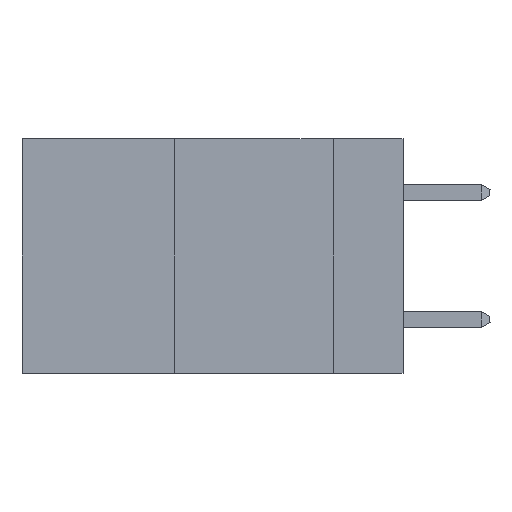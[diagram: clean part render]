
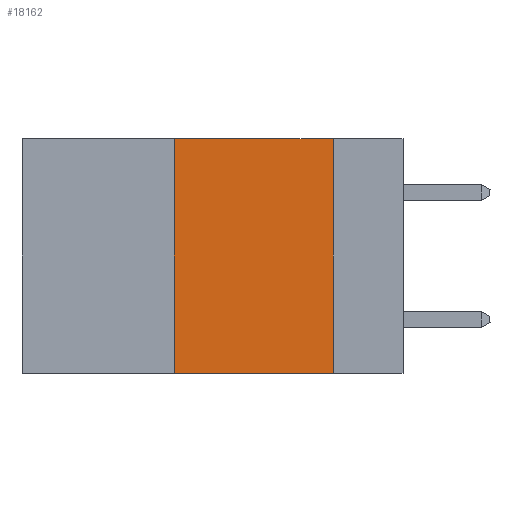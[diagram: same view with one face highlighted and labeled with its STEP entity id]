
A CAD part, left-side view. The second image highlights one B-rep face of the part: STEP entity #18162.
In plain terms, the highlighted planar face has unit normal (-1, 0, 0).
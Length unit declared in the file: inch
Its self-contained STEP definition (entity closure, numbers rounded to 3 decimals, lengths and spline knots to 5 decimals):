
#11 = VERTEX_POINT ( 'NONE', #24485 ) ;
#200 = VECTOR ( 'NONE', #6574, 39.37008 ) ;
#319 = DIRECTION ( 'NONE',  ( 0., -1., 0. ) ) ;
#517 = VECTOR ( 'NONE', #319, 39.37008 ) ;
#1247 = VERTEX_POINT ( 'NONE', #2486 ) ;
#2344 = DIRECTION ( 'NONE',  ( 0., -1., 0. ) ) ;
#2433 = CARTESIAN_POINT ( 'NONE',  ( 0., 0.6, -0.37 ) ) ;
#2486 = CARTESIAN_POINT ( 'NONE',  ( 0., 0.36, 0. ) ) ;
#3114 = LINE ( 'NONE', #2433, #20124 ) ;
#3671 = LINE ( 'NONE', #13528, #18319 ) ;
#3901 = DIRECTION ( 'NONE',  ( 0., 0., 1. ) ) ;
#4384 = VERTEX_POINT ( 'NONE', #10587 ) ;
#4588 = CARTESIAN_POINT ( 'NONE',  ( 0., 0.6, 0. ) ) ;
#4673 = EDGE_CURVE ( 'NONE', #23606, #1247, #3671, .T. ) ;
#5269 = LINE ( 'NONE', #14112, #200 ) ;
#6574 = DIRECTION ( 'NONE',  ( 0., 0., -1. ) ) ;
#10587 = CARTESIAN_POINT ( 'NONE',  ( 0., 0.11, -0.37 ) ) ;
#12683 = EDGE_CURVE ( 'NONE', #11, #4384, #5269, .T. ) ;
#13528 = CARTESIAN_POINT ( 'NONE',  ( 0., 0.36, 0. ) ) ;
#13600 = ORIENTED_EDGE ( 'NONE', *, *, #14189, .T. ) ;
#13747 = CARTESIAN_POINT ( 'NONE',  ( 0., 0.36, -0.37 ) ) ;
#14112 = CARTESIAN_POINT ( 'NONE',  ( 0., 0.11, 0. ) ) ;
#14121 = FACE_OUTER_BOUND ( 'NONE', #17262, .T. ) ;
#14189 = EDGE_CURVE ( 'NONE', #23606, #4384, #3114, .T. ) ;
#15703 = ORIENTED_EDGE ( 'NONE', *, *, #21966, .F. ) ;
#16755 = ORIENTED_EDGE ( 'NONE', *, *, #12683, .F. ) ;
#17262 = EDGE_LOOP ( 'NONE', ( #16755, #15703, #23046, #13600 ) ) ;
#17773 = DIRECTION ( 'NONE',  ( 1., 0., 0. ) ) ;
#17933 = DIRECTION ( 'NONE',  ( 0., 0., -1. ) ) ;
#18162 = ADVANCED_FACE ( 'NONE', ( #14121 ), #19528, .F. ) ;
#18319 = VECTOR ( 'NONE', #3901, 39.37008 ) ;
#19528 = PLANE ( 'NONE',  #22137 ) ;
#19603 = LINE ( 'NONE', #23049, #517 ) ;
#20124 = VECTOR ( 'NONE', #2344, 39.37008 ) ;
#21966 = EDGE_CURVE ( 'NONE', #1247, #11, #19603, .T. ) ;
#22137 = AXIS2_PLACEMENT_3D ( 'NONE', #4588, #17773, #17933 ) ;
#23046 = ORIENTED_EDGE ( 'NONE', *, *, #4673, .F. ) ;
#23049 = CARTESIAN_POINT ( 'NONE',  ( 0., 0.6, 0. ) ) ;
#23606 = VERTEX_POINT ( 'NONE', #13747 ) ;
#24485 = CARTESIAN_POINT ( 'NONE',  ( 0., 0.11, 0. ) ) ;
